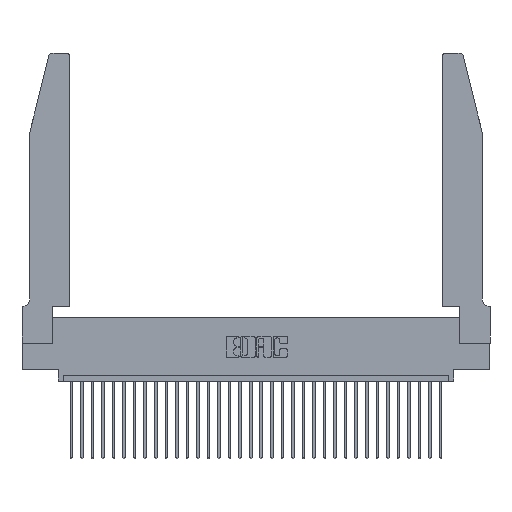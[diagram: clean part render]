
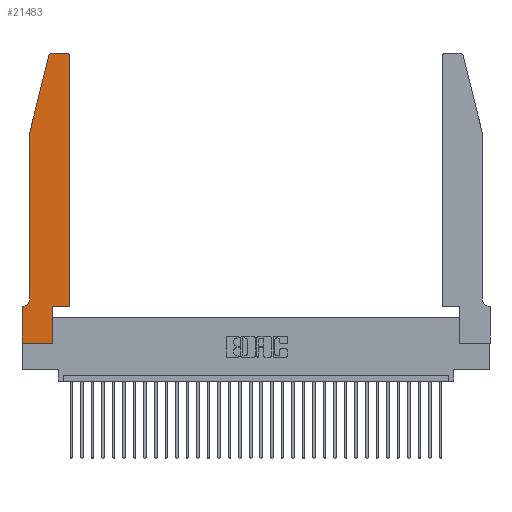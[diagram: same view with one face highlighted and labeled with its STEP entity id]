
A CAD part, top view. The second image highlights one B-rep face of the part: STEP entity #21483.
In plain terms, the highlighted planar face has unit normal (0, 0, 1).
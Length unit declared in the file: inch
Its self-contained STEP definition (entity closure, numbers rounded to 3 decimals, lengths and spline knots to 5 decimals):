
#533 = VERTEX_POINT ( 'NONE', #18986 ) ;
#553 = DIRECTION ( 'NONE',  ( -0.239, -0.971, 0. ) ) ;
#639 = VERTEX_POINT ( 'NONE', #15013 ) ;
#648 = VECTOR ( 'NONE', #1841, 39.37008 ) ;
#797 = EDGE_CURVE ( 'NONE', #14606, #26745, #12944, .T. ) ;
#1063 = LINE ( 'NONE', #11936, #648 ) ;
#1647 = VECTOR ( 'NONE', #553, 39.37008 ) ;
#1841 = DIRECTION ( 'NONE',  ( 1., 0., 0. ) ) ;
#1985 = DIRECTION ( 'NONE',  ( 1., 0., 0. ) ) ;
#2064 = VERTEX_POINT ( 'NONE', #6025 ) ;
#2081 = CARTESIAN_POINT ( 'NONE',  ( 0.0755, 0.35, 0.37 ) ) ;
#2229 = VECTOR ( 'NONE', #15870, 39.37008 ) ;
#2427 = CARTESIAN_POINT ( 'NONE',  ( 0.284, 2.72, 0.37 ) ) ;
#2592 = AXIS2_PLACEMENT_3D ( 'NONE', #17635, #17525, #22582 ) ;
#2836 = VERTEX_POINT ( 'NONE', #10013 ) ;
#3284 = EDGE_CURVE ( 'NONE', #13580, #22420, #15445, .T. ) ;
#3324 = CARTESIAN_POINT ( 'NONE',  ( 0.4505, 0.35, 0.37 ) ) ;
#4000 = ORIENTED_EDGE ( 'NONE', *, *, #6027, .T. ) ;
#4497 = ORIENTED_EDGE ( 'NONE', *, *, #25831, .T. ) ;
#5243 = ORIENTED_EDGE ( 'NONE', *, *, #18728, .T. ) ;
#5429 = CIRCLE ( 'NONE', #30005, 0.07 ) ;
#6025 = CARTESIAN_POINT ( 'NONE',  ( 0., 0.35, 0.37 ) ) ;
#6027 = EDGE_CURVE ( 'NONE', #19844, #31891, #12897, .T. ) ;
#6281 = VECTOR ( 'NONE', #7399, 39.37008 ) ;
#6442 = CARTESIAN_POINT ( 'NONE',  ( 0.25487, 2.72718, 0.37 ) ) ;
#7011 = DIRECTION ( 'NONE',  ( 0., 0., 1. ) ) ;
#7399 = DIRECTION ( 'NONE',  ( -1., 0., 0. ) ) ;
#7662 = PLANE ( 'NONE',  #2592 ) ;
#7708 = ORIENTED_EDGE ( 'NONE', *, *, #31158, .T. ) ;
#7849 = LINE ( 'NONE', #28390, #2229 ) ;
#8275 = AXIS2_PLACEMENT_3D ( 'NONE', #2427, #15256, #27574 ) ;
#9187 = CARTESIAN_POINT ( 'NONE',  ( 0.0055, 0.42, 0.37 ) ) ;
#9467 = CARTESIAN_POINT ( 'NONE',  ( 0.4205, 2.72, 0.37 ) ) ;
#9977 = ORIENTED_EDGE ( 'NONE', *, *, #11300, .T. ) ;
#10003 = VERTEX_POINT ( 'NONE', #20200 ) ;
#10013 = CARTESIAN_POINT ( 'NONE',  ( 0.2865, 0., 0.37 ) ) ;
#10410 = EDGE_LOOP ( 'NONE', ( #5243, #12250, #7708, #4000, #9977, #4497, #19226, #10548, #15471, #28003, #12914, #32574 ) ) ;
#10448 = CARTESIAN_POINT ( 'NONE',  ( 0.284, 2.75, 0.37 ) ) ;
#10548 = ORIENTED_EDGE ( 'NONE', *, *, #10620, .T. ) ;
#10620 = EDGE_CURVE ( 'NONE', #10003, #2836, #1063, .T. ) ;
#10812 = FACE_OUTER_BOUND ( 'NONE', #10410, .T. ) ;
#11238 = CARTESIAN_POINT ( 'NONE',  ( 0.2605, 2.75, 0.37 ) ) ;
#11300 = EDGE_CURVE ( 'NONE', #31891, #12604, #5429, .T. ) ;
#11936 = CARTESIAN_POINT ( 'NONE',  ( 0., 0., 0.37 ) ) ;
#12250 = ORIENTED_EDGE ( 'NONE', *, *, #3284, .T. ) ;
#12507 = CARTESIAN_POINT ( 'NONE',  ( 0.0055, 0.35, 0.37 ) ) ;
#12571 = LINE ( 'NONE', #15915, #24816 ) ;
#12604 = VERTEX_POINT ( 'NONE', #12507 ) ;
#12649 = CARTESIAN_POINT ( 'NONE',  ( 0.0755, 0.42, 0.37 ) ) ;
#12897 = LINE ( 'NONE', #31626, #26689 ) ;
#12914 = ORIENTED_EDGE ( 'NONE', *, *, #797, .T. ) ;
#12944 = LINE ( 'NONE', #3324, #18823 ) ;
#13217 = LINE ( 'NONE', #30677, #1647 ) ;
#13580 = VERTEX_POINT ( 'NONE', #10448 ) ;
#14606 = VERTEX_POINT ( 'NONE', #21676 ) ;
#14856 = CARTESIAN_POINT ( 'NONE',  ( 0.4505, 0.35, 0.37 ) ) ;
#15013 = CARTESIAN_POINT ( 'NONE',  ( 0.4205, 2.75, 0.37 ) ) ;
#15256 = DIRECTION ( 'NONE',  ( 0., 0., 1. ) ) ;
#15445 = CIRCLE ( 'NONE', #8275, 0.03 ) ;
#15471 = ORIENTED_EDGE ( 'NONE', *, *, #27157, .T. ) ;
#15870 = DIRECTION ( 'NONE',  ( 0., -1., 0. ) ) ;
#15915 = CARTESIAN_POINT ( 'NONE',  ( 0.2865, 0.35, 0.37 ) ) ;
#16016 = DIRECTION ( 'NONE',  ( 0., -1., 0. ) ) ;
#17525 = DIRECTION ( 'NONE',  ( 0., 0., 1. ) ) ;
#17635 = CARTESIAN_POINT ( 'NONE',  ( 0., 0.35, 0.37 ) ) ;
#18728 = EDGE_CURVE ( 'NONE', #639, #13580, #26798, .T. ) ;
#18823 = VECTOR ( 'NONE', #18898, 39.37008 ) ;
#18898 = DIRECTION ( 'NONE',  ( 0., 1., 0. ) ) ;
#18986 = CARTESIAN_POINT ( 'NONE',  ( 0.2865, 0.35, 0.37 ) ) ;
#19226 = ORIENTED_EDGE ( 'NONE', *, *, #26101, .T. ) ;
#19844 = VERTEX_POINT ( 'NONE', #24756 ) ;
#20141 = LINE ( 'NONE', #2081, #6281 ) ;
#20200 = CARTESIAN_POINT ( 'NONE',  ( 0., 0., 0.37 ) ) ;
#21125 = CIRCLE ( 'NONE', #27564, 0.03 ) ;
#21165 = DIRECTION ( 'NONE',  ( -1., 0., 0. ) ) ;
#21483 = ADVANCED_FACE ( 'NONE', ( #10812 ), #7662, .T. ) ;
#21676 = CARTESIAN_POINT ( 'NONE',  ( 0.4505, 0.35, 0.37 ) ) ;
#22131 = DIRECTION ( 'NONE',  ( 1., 0., 0. ) ) ;
#22336 = EDGE_CURVE ( 'NONE', #26745, #639, #21125, .T. ) ;
#22420 = VERTEX_POINT ( 'NONE', #6442 ) ;
#22582 = DIRECTION ( 'NONE',  ( 1., 0., 0. ) ) ;
#23076 = DIRECTION ( 'NONE',  ( 0., 1., 0. ) ) ;
#24047 = DIRECTION ( 'NONE',  ( 0., 0., -1. ) ) ;
#24756 = CARTESIAN_POINT ( 'NONE',  ( 0.0755, 2., 0.37 ) ) ;
#24816 = VECTOR ( 'NONE', #23076, 39.37008 ) ;
#25238 = VECTOR ( 'NONE', #21165, 39.37008 ) ;
#25831 = EDGE_CURVE ( 'NONE', #12604, #2064, #20141, .T. ) ;
#26101 = EDGE_CURVE ( 'NONE', #2064, #10003, #7849, .T. ) ;
#26689 = VECTOR ( 'NONE', #16016, 39.37008 ) ;
#26745 = VERTEX_POINT ( 'NONE', #28907 ) ;
#26798 = LINE ( 'NONE', #11238, #25238 ) ;
#27009 = DIRECTION ( 'NONE',  ( -1., 0., 0. ) ) ;
#27157 = EDGE_CURVE ( 'NONE', #2836, #533, #12571, .T. ) ;
#27538 = EDGE_CURVE ( 'NONE', #533, #14606, #31415, .T. ) ;
#27564 = AXIS2_PLACEMENT_3D ( 'NONE', #9467, #7011, #22131 ) ;
#27574 = DIRECTION ( 'NONE',  ( 1., 0., 0. ) ) ;
#28003 = ORIENTED_EDGE ( 'NONE', *, *, #27538, .T. ) ;
#28390 = CARTESIAN_POINT ( 'NONE',  ( 0., 0., 0.37 ) ) ;
#28907 = CARTESIAN_POINT ( 'NONE',  ( 0.4505, 2.72, 0.37 ) ) ;
#30005 = AXIS2_PLACEMENT_3D ( 'NONE', #9187, #24047, #27009 ) ;
#30677 = CARTESIAN_POINT ( 'NONE',  ( 0.0755, 2., 0.37 ) ) ;
#31158 = EDGE_CURVE ( 'NONE', #22420, #19844, #13217, .T. ) ;
#31415 = LINE ( 'NONE', #14856, #32620 ) ;
#31626 = CARTESIAN_POINT ( 'NONE',  ( 0.0755, 2., 0.37 ) ) ;
#31891 = VERTEX_POINT ( 'NONE', #12649 ) ;
#32574 = ORIENTED_EDGE ( 'NONE', *, *, #22336, .T. ) ;
#32620 = VECTOR ( 'NONE', #1985, 39.37008 ) ;
